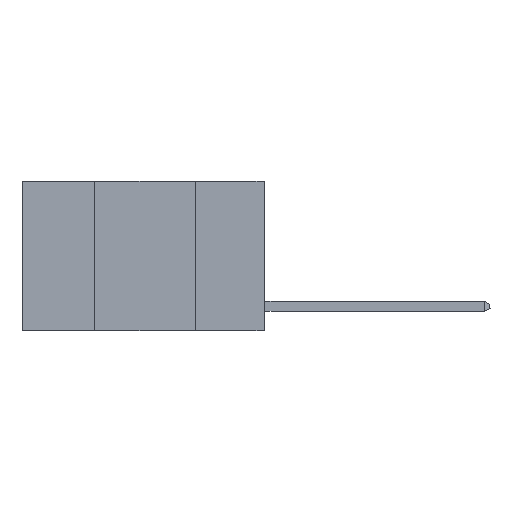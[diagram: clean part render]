
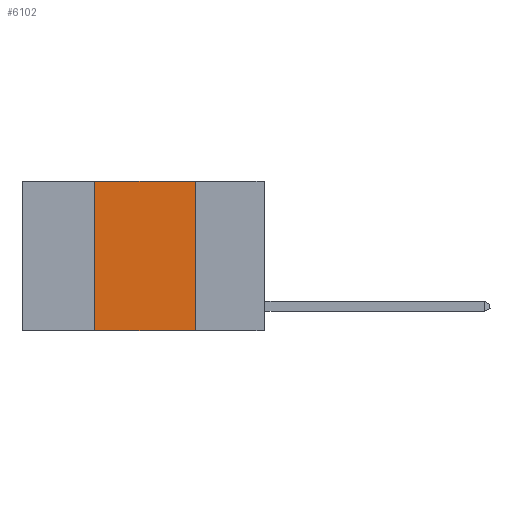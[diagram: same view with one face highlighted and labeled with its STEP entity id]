
A CAD part, left-side view. The second image highlights one B-rep face of the part: STEP entity #6102.
In plain terms, the highlighted planar face has unit normal (-1, 0, 0).
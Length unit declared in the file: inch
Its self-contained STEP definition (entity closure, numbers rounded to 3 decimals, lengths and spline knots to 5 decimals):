
#100 = LINE ( 'NONE', #4495, #7088 ) ;
#112 = VECTOR ( 'NONE', #241, 39.37008 ) ;
#214 = CARTESIAN_POINT ( 'NONE',  ( 0., 0.6, 0. ) ) ;
#241 = DIRECTION ( 'NONE',  ( 0., -1., 0. ) ) ;
#587 = CARTESIAN_POINT ( 'NONE',  ( 0., 0.17, 0. ) ) ;
#753 = PLANE ( 'NONE',  #7828 ) ;
#1035 = DIRECTION ( 'NONE',  ( 0., 0., -1. ) ) ;
#1155 = CARTESIAN_POINT ( 'NONE',  ( 0., 0.17, -0.37 ) ) ;
#1181 = EDGE_CURVE ( 'NONE', #8148, #1511, #5920, .T. ) ;
#1409 = DIRECTION ( 'NONE',  ( 1., 0., 0. ) ) ;
#1511 = VERTEX_POINT ( 'NONE', #1155 ) ;
#1835 = CARTESIAN_POINT ( 'NONE',  ( 0., 0.17, 0. ) ) ;
#1900 = ORIENTED_EDGE ( 'NONE', *, *, #1181, .F. ) ;
#1991 = CARTESIAN_POINT ( 'NONE',  ( 0., 0.42, -0.37 ) ) ;
#2078 = VERTEX_POINT ( 'NONE', #2348 ) ;
#2312 = FACE_OUTER_BOUND ( 'NONE', #5315, .T. ) ;
#2348 = CARTESIAN_POINT ( 'NONE',  ( 0., 0.42, 0. ) ) ;
#2657 = DIRECTION ( 'NONE',  ( 0., -1., 0. ) ) ;
#2774 = ORIENTED_EDGE ( 'NONE', *, *, #4090, .F. ) ;
#2980 = ORIENTED_EDGE ( 'NONE', *, *, #7620, .F. ) ;
#4090 = EDGE_CURVE ( 'NONE', #6659, #2078, #100, .T. ) ;
#4123 = DIRECTION ( 'NONE',  ( 0., 0., 1. ) ) ;
#4125 = VECTOR ( 'NONE', #1035, 39.37008 ) ;
#4495 = CARTESIAN_POINT ( 'NONE',  ( 0., 0.42, 0. ) ) ;
#4893 = VECTOR ( 'NONE', #2657, 39.37008 ) ;
#5016 = ORIENTED_EDGE ( 'NONE', *, *, #8647, .T. ) ;
#5315 = EDGE_LOOP ( 'NONE', ( #1900, #2980, #2774, #5016 ) ) ;
#5920 = LINE ( 'NONE', #1835, #4125 ) ;
#6063 = DIRECTION ( 'NONE',  ( 0., 0., -1. ) ) ;
#6102 = ADVANCED_FACE ( 'NONE', ( #2312 ), #753, .F. ) ;
#6659 = VERTEX_POINT ( 'NONE', #1991 ) ;
#6693 = CARTESIAN_POINT ( 'NONE',  ( 0., 0.6, -0.37 ) ) ;
#7088 = VECTOR ( 'NONE', #4123, 39.37008 ) ;
#7296 = LINE ( 'NONE', #214, #112 ) ;
#7408 = CARTESIAN_POINT ( 'NONE',  ( 0., 0.6, 0. ) ) ;
#7620 = EDGE_CURVE ( 'NONE', #2078, #8148, #7296, .T. ) ;
#7828 = AXIS2_PLACEMENT_3D ( 'NONE', #7408, #1409, #6063 ) ;
#8073 = LINE ( 'NONE', #6693, #4893 ) ;
#8148 = VERTEX_POINT ( 'NONE', #587 ) ;
#8647 = EDGE_CURVE ( 'NONE', #6659, #1511, #8073, .T. ) ;
